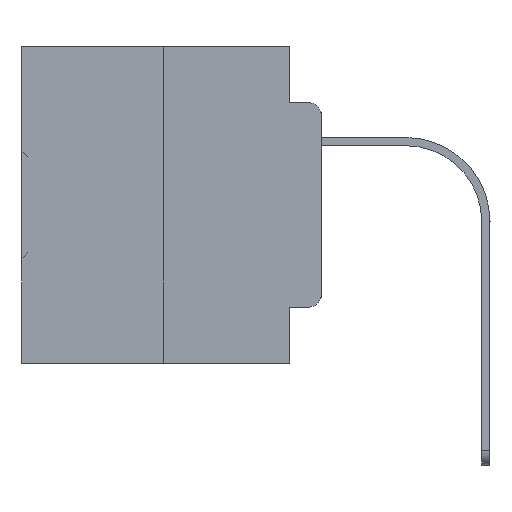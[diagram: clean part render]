
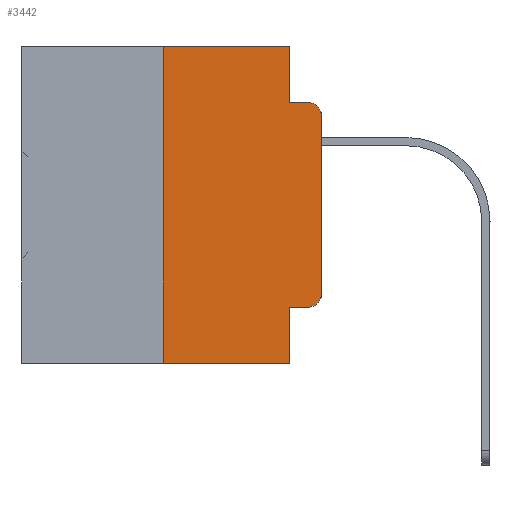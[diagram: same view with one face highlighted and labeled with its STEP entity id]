
A CAD part, left-side view. The second image highlights one B-rep face of the part: STEP entity #3442.
In plain terms, the highlighted planar face has unit normal (-1, 0, 0).
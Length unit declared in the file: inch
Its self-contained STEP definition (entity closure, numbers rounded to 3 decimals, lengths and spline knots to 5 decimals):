
#569 = EDGE_CURVE ( 'NONE', #20599, #11035, #2884, .T. ) ;
#1418 = LINE ( 'NONE', #3937, #32409 ) ;
#1654 = EDGE_CURVE ( 'NONE', #13742, #7034, #34957, .T. ) ;
#2136 = CARTESIAN_POINT ( 'NONE',  ( 0., 0.473, 0. ) ) ;
#2884 = LINE ( 'NONE', #24693, #19592 ) ;
#3110 = DIRECTION ( 'NONE',  ( 0., 0., 1. ) ) ;
#3199 = DIRECTION ( 'NONE',  ( 0., 0., -1. ) ) ;
#3257 = ORIENTED_EDGE ( 'NONE', *, *, #1654, .F. ) ;
#3442 = ADVANCED_FACE ( 'NONE', ( #30196 ), #22145, .F. ) ;
#3814 = VECTOR ( 'NONE', #7711, 39.37008 ) ;
#3937 = CARTESIAN_POINT ( 'NONE',  ( 0., 0.051, -0.0885 ) ) ;
#5257 = CARTESIAN_POINT ( 'NONE',  ( 0., 0.25, 0. ) ) ;
#5505 = AXIS2_PLACEMENT_3D ( 'NONE', #22267, #21574, #29980 ) ;
#6520 = EDGE_CURVE ( 'NONE', #23758, #7034, #10127, .T. ) ;
#6867 = DIRECTION ( 'NONE',  ( -1., 0., 0. ) ) ;
#7034 = VERTEX_POINT ( 'NONE', #8300 ) ;
#7221 = EDGE_CURVE ( 'NONE', #20355, #28460, #1418, .T. ) ;
#7280 = CARTESIAN_POINT ( 'NONE',  ( 0., 0.473, -0.5 ) ) ;
#7711 = DIRECTION ( 'NONE',  ( 0., -1., 0. ) ) ;
#7984 = CARTESIAN_POINT ( 'NONE',  ( 0., 0.051, 0. ) ) ;
#8300 = CARTESIAN_POINT ( 'NONE',  ( 0., 0.051, -0.5 ) ) ;
#8565 = CARTESIAN_POINT ( 'NONE',  ( 0., 0.473, 0. ) ) ;
#9096 = VECTOR ( 'NONE', #25062, 39.37008 ) ;
#9275 = CARTESIAN_POINT ( 'NONE',  ( 0., 0.02, -0.0885 ) ) ;
#10013 = DIRECTION ( 'NONE',  ( 0., -1., 0. ) ) ;
#10127 = LINE ( 'NONE', #7280, #15901 ) ;
#10257 = ORIENTED_EDGE ( 'NONE', *, *, #20889, .T. ) ;
#11035 = VERTEX_POINT ( 'NONE', #16724 ) ;
#12598 = VERTEX_POINT ( 'NONE', #24228 ) ;
#12635 = CARTESIAN_POINT ( 'NONE',  ( 0., 0.25, -0.5 ) ) ;
#12666 = LINE ( 'NONE', #20721, #28272 ) ;
#13742 = VERTEX_POINT ( 'NONE', #17199 ) ;
#13785 = DIRECTION ( 'NONE',  ( 0., 0., 1. ) ) ;
#13977 = AXIS2_PLACEMENT_3D ( 'NONE', #8565, #22483, #3199 ) ;
#15176 = CIRCLE ( 'NONE', #5505, 0.02 ) ;
#15643 = VERTEX_POINT ( 'NONE', #34685 ) ;
#15780 = DIRECTION ( 'NONE',  ( 0., 0., -1. ) ) ;
#15901 = VECTOR ( 'NONE', #18536, 39.37008 ) ;
#16613 = ORIENTED_EDGE ( 'NONE', *, *, #33483, .F. ) ;
#16651 = LINE ( 'NONE', #19703, #9096 ) ;
#16724 = CARTESIAN_POINT ( 'NONE',  ( 0., 0., -0.1085 ) ) ;
#16877 = EDGE_CURVE ( 'NONE', #17073, #20599, #21897, .T. ) ;
#17073 = VERTEX_POINT ( 'NONE', #30903 ) ;
#17199 = CARTESIAN_POINT ( 'NONE',  ( 0., 0.051, -0.4115 ) ) ;
#18536 = DIRECTION ( 'NONE',  ( 0., -1., 0. ) ) ;
#19592 = VECTOR ( 'NONE', #13785, 39.37008 ) ;
#19703 = CARTESIAN_POINT ( 'NONE',  ( 0., 0.051, 0. ) ) ;
#20227 = EDGE_CURVE ( 'NONE', #13742, #17073, #12666, .T. ) ;
#20355 = VERTEX_POINT ( 'NONE', #35216 ) ;
#20599 = VERTEX_POINT ( 'NONE', #26388 ) ;
#20721 = CARTESIAN_POINT ( 'NONE',  ( 0., 0.051, -0.4115 ) ) ;
#20889 = EDGE_CURVE ( 'NONE', #11035, #28460, #15176, .T. ) ;
#21574 = DIRECTION ( 'NONE',  ( -1., 0., 0. ) ) ;
#21605 = ORIENTED_EDGE ( 'NONE', *, *, #24567, .F. ) ;
#21897 = CIRCLE ( 'NONE', #27039, 0.02 ) ;
#22145 = PLANE ( 'NONE',  #13977 ) ;
#22267 = CARTESIAN_POINT ( 'NONE',  ( 0., 0.02, -0.1085 ) ) ;
#22483 = DIRECTION ( 'NONE',  ( 1., 0., 0. ) ) ;
#22564 = ORIENTED_EDGE ( 'NONE', *, *, #7221, .F. ) ;
#22982 = VECTOR ( 'NONE', #29608, 39.37008 ) ;
#23505 = ORIENTED_EDGE ( 'NONE', *, *, #20227, .T. ) ;
#23758 = VERTEX_POINT ( 'NONE', #12635 ) ;
#24228 = CARTESIAN_POINT ( 'NONE',  ( 0., 0.25, 0. ) ) ;
#24567 = EDGE_CURVE ( 'NONE', #12598, #15643, #32004, .T. ) ;
#24693 = CARTESIAN_POINT ( 'NONE',  ( 0., 0., 0. ) ) ;
#25062 = DIRECTION ( 'NONE',  ( 0., 0., -1. ) ) ;
#26269 = DIRECTION ( 'NONE',  ( 0., -1., 0. ) ) ;
#26388 = CARTESIAN_POINT ( 'NONE',  ( 0., 0., -0.3915 ) ) ;
#27039 = AXIS2_PLACEMENT_3D ( 'NONE', #34034, #6867, #15780 ) ;
#28272 = VECTOR ( 'NONE', #26269, 39.37008 ) ;
#28460 = VERTEX_POINT ( 'NONE', #9275 ) ;
#29557 = ORIENTED_EDGE ( 'NONE', *, *, #569, .T. ) ;
#29608 = DIRECTION ( 'NONE',  ( 0., 0., -1. ) ) ;
#29686 = ORIENTED_EDGE ( 'NONE', *, *, #31659, .F. ) ;
#29754 = LINE ( 'NONE', #5257, #33631 ) ;
#29980 = DIRECTION ( 'NONE',  ( 0., 0., -1. ) ) ;
#30051 = ORIENTED_EDGE ( 'NONE', *, *, #6520, .T. ) ;
#30196 = FACE_OUTER_BOUND ( 'NONE', #35288, .T. ) ;
#30903 = CARTESIAN_POINT ( 'NONE',  ( 0., 0.02, -0.4115 ) ) ;
#31659 = EDGE_CURVE ( 'NONE', #15643, #20355, #16651, .T. ) ;
#31973 = ORIENTED_EDGE ( 'NONE', *, *, #16877, .T. ) ;
#32004 = LINE ( 'NONE', #2136, #3814 ) ;
#32409 = VECTOR ( 'NONE', #10013, 39.37008 ) ;
#33483 = EDGE_CURVE ( 'NONE', #23758, #12598, #29754, .T. ) ;
#33631 = VECTOR ( 'NONE', #3110, 39.37008 ) ;
#34034 = CARTESIAN_POINT ( 'NONE',  ( 0., 0.02, -0.3915 ) ) ;
#34685 = CARTESIAN_POINT ( 'NONE',  ( 0., 0.051, 0. ) ) ;
#34957 = LINE ( 'NONE', #7984, #22982 ) ;
#35216 = CARTESIAN_POINT ( 'NONE',  ( 0., 0.051, -0.0885 ) ) ;
#35288 = EDGE_LOOP ( 'NONE', ( #29557, #10257, #22564, #29686, #21605, #16613, #30051, #3257, #23505, #31973 ) ) ;
